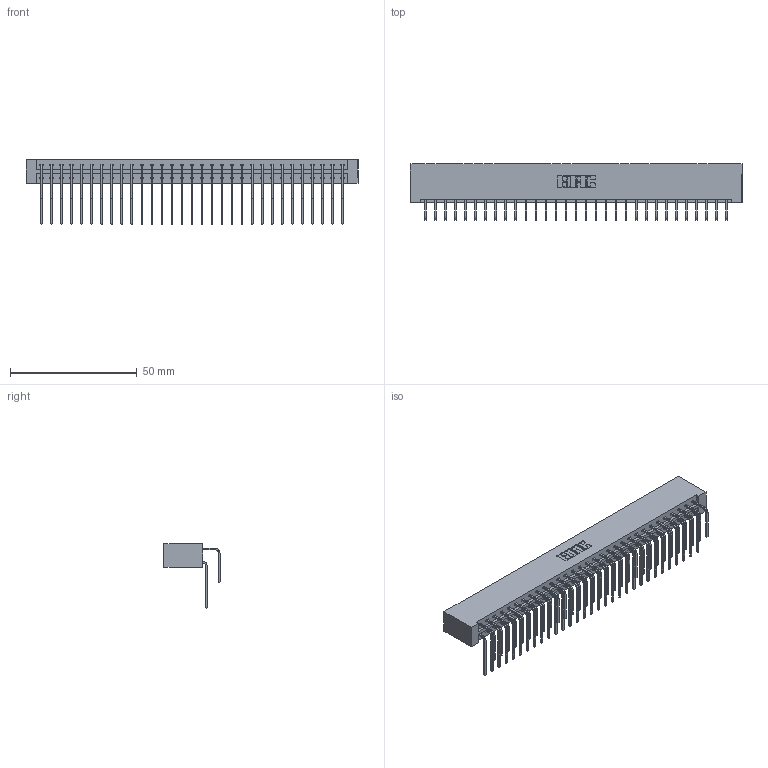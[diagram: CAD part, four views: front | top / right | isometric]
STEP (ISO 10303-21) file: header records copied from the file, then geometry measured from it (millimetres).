
FILE_DESCRIPTION (( 'STEP AP203' ), '1' );
FILE_NAME ('333-062-558-201.STEP', '2018-08-04T09:01:50', ( '' ), ( '' ), 'SwSTEP 2.0', 'SolidWorks 2016', '' );
FILE_SCHEMA (( 'CONFIG_CONTROL_DESIGN' ));
Length unit declared in the file: inch
Products named in the file (4): 345-292-001_558 Tail - 2; 333-062-558-201; 333 Part_Lugless; 345-292-001_558 559 Tail - 1
Assembly tree (63 placements, depth 2):
  333-062-558-201
    333 Part_Lugless
    345-292-001_558 559 Tail - 1  x31
    345-292-001_558 Tail - 2  x31
Bounding box: 131.09 x 22.17 x 25.53 mm (x, y, z)
Volume: 14270.5 mm3; surface area: 18559 mm2
Topology: 63 solids, 63 shells, 3454 faces, 10269 edges, 6762 vertices
Faces by surface type: plane 2422, cylinder 1032
Entity records: 22873 total; most frequent: CARTESIAN_POINT 3853, ORIENTED_EDGE 3738, DIRECTION 3285, EDGE_CURVE 1869, LINE 1709, VECTOR 1709, VERTEX_POINT 1242, AXIS2_PLACEMENT_3D 788
